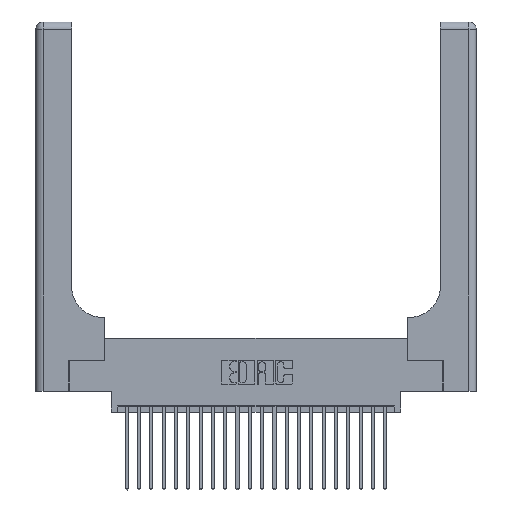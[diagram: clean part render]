
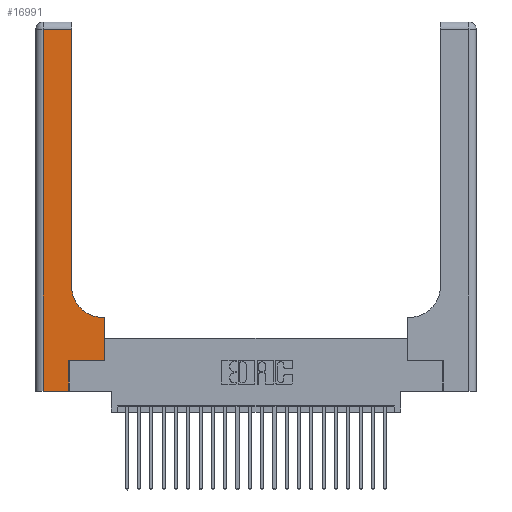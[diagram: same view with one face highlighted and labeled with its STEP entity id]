
A CAD part, top view. The second image highlights one B-rep face of the part: STEP entity #16991.
In plain terms, the highlighted planar face has unit normal (0, 0, 1).
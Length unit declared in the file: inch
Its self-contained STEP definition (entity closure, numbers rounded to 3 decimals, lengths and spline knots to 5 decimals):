
#528 = VECTOR ( 'NONE', #17226, 39.37008 ) ;
#575 = CARTESIAN_POINT ( 'NONE',  ( 0.2915, 2.94, 0.37 ) ) ;
#578 = PLANE ( 'NONE',  #18245 ) ;
#713 = FACE_OUTER_BOUND ( 'NONE', #1214, .T. ) ;
#824 = VERTEX_POINT ( 'NONE', #5884 ) ;
#946 = CARTESIAN_POINT ( 'NONE',  ( 0.06, 2.94, 0.37 ) ) ;
#1214 = EDGE_LOOP ( 'NONE', ( #9697, #17049, #15419, #2678, #16907, #4828, #6877, #16718, #21640 ) ) ;
#1376 = CARTESIAN_POINT ( 'NONE',  ( 0.06, 3., 0.37 ) ) ;
#1507 = CARTESIAN_POINT ( 'NONE',  ( 0.269, 0.25, 0.37 ) ) ;
#1674 = LINE ( 'NONE', #3525, #19121 ) ;
#1784 = DIRECTION ( 'NONE',  ( 0., 1., 0. ) ) ;
#2317 = EDGE_CURVE ( 'NONE', #16483, #16218, #18565, .T. ) ;
#2408 = DIRECTION ( 'NONE',  ( 0., 0., -1. ) ) ;
#2496 = DIRECTION ( 'NONE',  ( 0., 1., 0. ) ) ;
#2678 = ORIENTED_EDGE ( 'NONE', *, *, #22448, .T. ) ;
#3395 = DIRECTION ( 'NONE',  ( 1., 0., 0. ) ) ;
#3525 = CARTESIAN_POINT ( 'NONE',  ( 0., 2.94, 0.37 ) ) ;
#4168 = CARTESIAN_POINT ( 'NONE',  ( 0.5415, 0.6, 0.37 ) ) ;
#4643 = CARTESIAN_POINT ( 'NONE',  ( 0.2915, 0.85, 0.37 ) ) ;
#4828 = ORIENTED_EDGE ( 'NONE', *, *, #7625, .T. ) ;
#5119 = LINE ( 'NONE', #17484, #528 ) ;
#5663 = DIRECTION ( 'NONE',  ( 0., 1., 0. ) ) ;
#5884 = CARTESIAN_POINT ( 'NONE',  ( 0.5585, 0.6, 0.37 ) ) ;
#6279 = DIRECTION ( 'NONE',  ( 1., 0., 0. ) ) ;
#6565 = CARTESIAN_POINT ( 'NONE',  ( 0., 3., 0.37 ) ) ;
#6877 = ORIENTED_EDGE ( 'NONE', *, *, #15221, .T. ) ;
#7278 = VECTOR ( 'NONE', #24705, 39.37008 ) ;
#7369 = AXIS2_PLACEMENT_3D ( 'NONE', #19793, #2408, #6279 ) ;
#7491 = VERTEX_POINT ( 'NONE', #4168 ) ;
#7625 = EDGE_CURVE ( 'NONE', #23617, #20433, #12844, .T. ) ;
#7831 = VECTOR ( 'NONE', #21284, 39.37008 ) ;
#7888 = CARTESIAN_POINT ( 'NONE',  ( 0.5585, 0.25, 0.37 ) ) ;
#7938 = VECTOR ( 'NONE', #3395, 39.37008 ) ;
#9446 = DIRECTION ( 'NONE',  ( -1., 0., 0. ) ) ;
#9697 = ORIENTED_EDGE ( 'NONE', *, *, #14307, .T. ) ;
#9906 = CARTESIAN_POINT ( 'NONE',  ( 0.2915, 3., 0.37 ) ) ;
#11531 = LINE ( 'NONE', #23408, #12136 ) ;
#12136 = VECTOR ( 'NONE', #1784, 39.37008 ) ;
#12368 = CIRCLE ( 'NONE', #7369, 0.25 ) ;
#12428 = VECTOR ( 'NONE', #5663, 39.37008 ) ;
#12844 = LINE ( 'NONE', #22486, #7938 ) ;
#14155 = DIRECTION ( 'NONE',  ( -1., 0., 0. ) ) ;
#14307 = EDGE_CURVE ( 'NONE', #17643, #14699, #15970, .T. ) ;
#14699 = VERTEX_POINT ( 'NONE', #575 ) ;
#15221 = EDGE_CURVE ( 'NONE', #20433, #824, #19479, .T. ) ;
#15419 = ORIENTED_EDGE ( 'NONE', *, *, #2317, .T. ) ;
#15477 = EDGE_CURVE ( 'NONE', #14699, #16483, #1674, .T. ) ;
#15711 = EDGE_CURVE ( 'NONE', #7491, #17643, #12368, .T. ) ;
#15970 = LINE ( 'NONE', #9906, #21504 ) ;
#16218 = VERTEX_POINT ( 'NONE', #19589 ) ;
#16483 = VERTEX_POINT ( 'NONE', #946 ) ;
#16718 = ORIENTED_EDGE ( 'NONE', *, *, #21801, .T. ) ;
#16907 = ORIENTED_EDGE ( 'NONE', *, *, #20984, .T. ) ;
#16991 = ADVANCED_FACE ( 'NONE', ( #713 ), #578, .F. ) ;
#17049 = ORIENTED_EDGE ( 'NONE', *, *, #15477, .T. ) ;
#17226 = DIRECTION ( 'NONE',  ( 1., 0., 0. ) ) ;
#17352 = CARTESIAN_POINT ( 'NONE',  ( 0.5585, 0.25, 0.37 ) ) ;
#17484 = CARTESIAN_POINT ( 'NONE',  ( 0., 0., 0.37 ) ) ;
#17589 = CARTESIAN_POINT ( 'NONE',  ( 0.269, 0., 0.37 ) ) ;
#17643 = VERTEX_POINT ( 'NONE', #4643 ) ;
#18245 = AXIS2_PLACEMENT_3D ( 'NONE', #6565, #19990, #14155 ) ;
#18565 = LINE ( 'NONE', #1376, #7278 ) ;
#19121 = VECTOR ( 'NONE', #9446, 39.37008 ) ;
#19310 = CARTESIAN_POINT ( 'NONE',  ( 0.2915, 0.6, 0.37 ) ) ;
#19455 = LINE ( 'NONE', #19310, #7831 ) ;
#19479 = LINE ( 'NONE', #17352, #12428 ) ;
#19589 = CARTESIAN_POINT ( 'NONE',  ( 0.06, 0., 0.37 ) ) ;
#19793 = CARTESIAN_POINT ( 'NONE',  ( 0.5415, 0.85, 0.37 ) ) ;
#19990 = DIRECTION ( 'NONE',  ( 0., 0., -1. ) ) ;
#20433 = VERTEX_POINT ( 'NONE', #7888 ) ;
#20984 = EDGE_CURVE ( 'NONE', #23784, #23617, #11531, .T. ) ;
#21284 = DIRECTION ( 'NONE',  ( -1., 0., 0. ) ) ;
#21504 = VECTOR ( 'NONE', #2496, 39.37008 ) ;
#21640 = ORIENTED_EDGE ( 'NONE', *, *, #15711, .T. ) ;
#21801 = EDGE_CURVE ( 'NONE', #824, #7491, #19455, .T. ) ;
#22448 = EDGE_CURVE ( 'NONE', #16218, #23784, #5119, .T. ) ;
#22486 = CARTESIAN_POINT ( 'NONE',  ( 0.269, 0.25, 0.37 ) ) ;
#23408 = CARTESIAN_POINT ( 'NONE',  ( 0.269, 0., 0.37 ) ) ;
#23617 = VERTEX_POINT ( 'NONE', #1507 ) ;
#23784 = VERTEX_POINT ( 'NONE', #17589 ) ;
#24705 = DIRECTION ( 'NONE',  ( 0., -1., 0. ) ) ;
